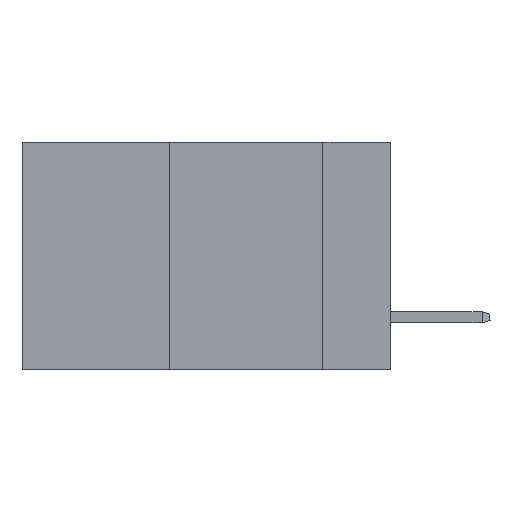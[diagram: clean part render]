
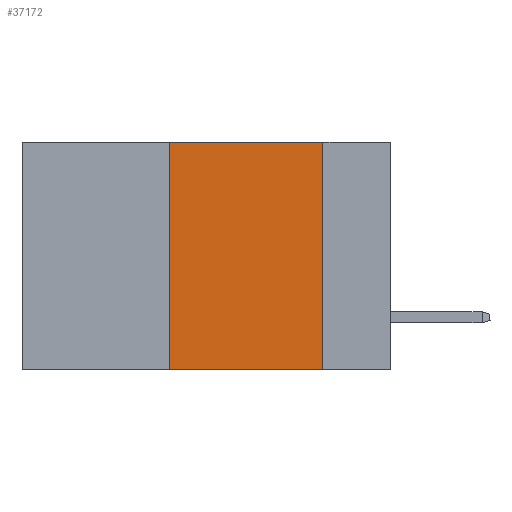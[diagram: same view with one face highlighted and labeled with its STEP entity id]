
A CAD part, left-side view. The second image highlights one B-rep face of the part: STEP entity #37172.
In plain terms, the highlighted planar face has unit normal (-1, 0, 0).
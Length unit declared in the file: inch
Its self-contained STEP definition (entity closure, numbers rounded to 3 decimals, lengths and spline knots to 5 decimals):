
#331 = ORIENTED_EDGE ( 'NONE', *, *, #15545, .F. ) ;
#478 = LINE ( 'NONE', #39910, #27932 ) ;
#2062 = CARTESIAN_POINT ( 'NONE',  ( 0., 0.36, 0. ) ) ;
#4963 = VECTOR ( 'NONE', #44010, 39.37008 ) ;
#4989 = CARTESIAN_POINT ( 'NONE',  ( 0., 0.6, -0.37 ) ) ;
#6408 = CARTESIAN_POINT ( 'NONE',  ( 0., 0.36, -0.37 ) ) ;
#7514 = DIRECTION ( 'NONE',  ( 0., -1., 0. ) ) ;
#8246 = AXIS2_PLACEMENT_3D ( 'NONE', #30589, #32697, #46367 ) ;
#8549 = ORIENTED_EDGE ( 'NONE', *, *, #45603, .F. ) ;
#10716 = VECTOR ( 'NONE', #7514, 39.37008 ) ;
#13948 = ORIENTED_EDGE ( 'NONE', *, *, #17908, .T. ) ;
#15545 = EDGE_CURVE ( 'NONE', #23463, #39002, #20936, .T. ) ;
#15990 = CARTESIAN_POINT ( 'NONE',  ( 0., 0.11, 0. ) ) ;
#17908 = EDGE_CURVE ( 'NONE', #38414, #29569, #50022, .T. ) ;
#18251 = LINE ( 'NONE', #46182, #36436 ) ;
#20936 = LINE ( 'NONE', #45828, #10716 ) ;
#23463 = VERTEX_POINT ( 'NONE', #2062 ) ;
#27932 = VECTOR ( 'NONE', #40244, 39.37008 ) ;
#29095 = EDGE_CURVE ( 'NONE', #39002, #29569, #18251, .T. ) ;
#29569 = VERTEX_POINT ( 'NONE', #31095 ) ;
#30589 = CARTESIAN_POINT ( 'NONE',  ( 0., 0.6, 0. ) ) ;
#31095 = CARTESIAN_POINT ( 'NONE',  ( 0., 0.11, -0.37 ) ) ;
#32697 = DIRECTION ( 'NONE',  ( 1., 0., 0. ) ) ;
#33645 = PLANE ( 'NONE',  #8246 ) ;
#34866 = DIRECTION ( 'NONE',  ( 0., 0., -1. ) ) ;
#36436 = VECTOR ( 'NONE', #34866, 39.37008 ) ;
#37172 = ADVANCED_FACE ( 'NONE', ( #47721 ), #33645, .F. ) ;
#38414 = VERTEX_POINT ( 'NONE', #6408 ) ;
#39002 = VERTEX_POINT ( 'NONE', #15990 ) ;
#39910 = CARTESIAN_POINT ( 'NONE',  ( 0., 0.36, 0. ) ) ;
#40244 = DIRECTION ( 'NONE',  ( 0., 0., 1. ) ) ;
#44010 = DIRECTION ( 'NONE',  ( 0., -1., 0. ) ) ;
#45603 = EDGE_CURVE ( 'NONE', #38414, #23463, #478, .T. ) ;
#45828 = CARTESIAN_POINT ( 'NONE',  ( 0., 0.6, 0. ) ) ;
#46182 = CARTESIAN_POINT ( 'NONE',  ( 0., 0.11, 0. ) ) ;
#46367 = DIRECTION ( 'NONE',  ( 0., 0., -1. ) ) ;
#46952 = EDGE_LOOP ( 'NONE', ( #50205, #331, #8549, #13948 ) ) ;
#47721 = FACE_OUTER_BOUND ( 'NONE', #46952, .T. ) ;
#50022 = LINE ( 'NONE', #4989, #4963 ) ;
#50205 = ORIENTED_EDGE ( 'NONE', *, *, #29095, .F. ) ;
